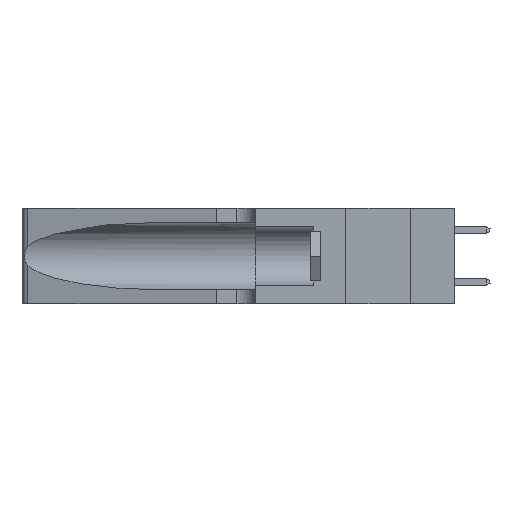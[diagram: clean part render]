
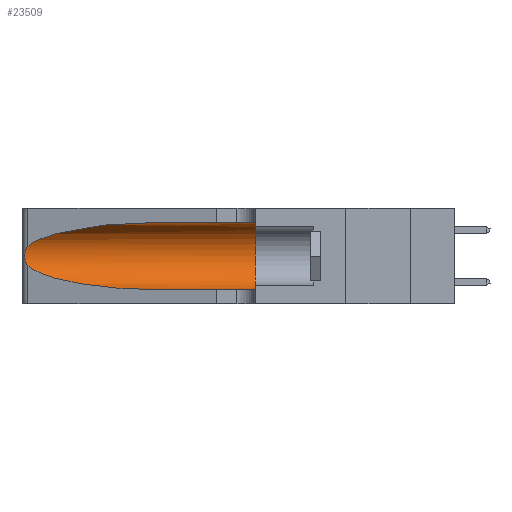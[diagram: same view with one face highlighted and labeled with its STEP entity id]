
A CAD part, left-side view. The second image highlights one B-rep face of the part: STEP entity #23509.
In plain terms, the highlighted cylindrical face has radius 3.308 mm (diameter 6.617 mm), a partial arc.
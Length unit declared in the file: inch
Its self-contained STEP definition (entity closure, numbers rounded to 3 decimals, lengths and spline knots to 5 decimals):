
#267 = VERTEX_POINT ( 'NONE', #5680 ) ;
#378 = VERTEX_POINT ( 'NONE', #12688 ) ;
#407 = CARTESIAN_POINT ( 'NONE',  ( 0.1305, 1.61858, 0.05475 ) ) ;
#580 = DIRECTION ( 'NONE',  ( 0., -1., 0. ) ) ;
#1451 = VERTEX_POINT ( 'NONE', #7885 ) ;
#1627 = CARTESIAN_POINT ( 'NONE',  ( 0.26075, 1.23896, 0.178 ) ) ;
#1999 =( BOUNDED_CURVE ( )  B_SPLINE_CURVE ( 3, ( #27865, #8334, #4212, #28052 ),
 .UNSPECIFIED., .F., .F. ) 
 B_SPLINE_CURVE_WITH_KNOTS ( ( 4, 4 ),
 ( 3.44316, 4.71239 ),
 .UNSPECIFIED. ) 
 CURVE ( )  GEOMETRIC_REPRESENTATION_ITEM ( )  RATIONAL_B_SPLINE_CURVE ( ( 1., 0.87, 0.87, 1. ) ) 
 REPRESENTATION_ITEM ( '' )  );
#2007 = CARTESIAN_POINT ( 'NONE',  ( 0.25639, 1.23184, 0.21858 ) ) ;
#2326 = DIRECTION ( 'NONE',  ( 0., 0., 1. ) ) ;
#2398 = LINE ( 'NONE', #3298, #26205 ) ;
#3022 = EDGE_CURVE ( 'NONE', #267, #16751, #1999, .T. ) ;
#3033 = EDGE_CURVE ( 'NONE', #16982, #267, #9717, .T. ) ;
#3298 = CARTESIAN_POINT ( 'NONE',  ( 0.1305, 1.61858, 0.31525 ) ) ;
#3930 = CARTESIAN_POINT ( 'NONE',  ( 0.25487, 1.22718, 0.14631 ) ) ;
#4212 = CARTESIAN_POINT ( 'NONE',  ( 0.18966, 0.96281, 0.05475 ) ) ;
#5383 = DIRECTION ( 'NONE',  ( 0., -1., 0. ) ) ;
#5680 = CARTESIAN_POINT ( 'NONE',  ( 0.25487, 1.22718, 0.14631 ) ) ;
#5920 = ORIENTED_EDGE ( 'NONE', *, *, #3022, .T. ) ;
#6170 = VERTEX_POINT ( 'NONE', #8930 ) ;
#6733 = CYLINDRICAL_SURFACE ( 'NONE', #8055, 0.13025 ) ;
#7602 =( BOUNDED_CURVE ( )  B_SPLINE_CURVE ( 3, ( #14610, #16617, #25393, #14525 ),
 .UNSPECIFIED., .F., .F. ) 
 B_SPLINE_CURVE_WITH_KNOTS ( ( 4, 4 ),
 ( 1.5708, 2.84003 ),
 .UNSPECIFIED. ) 
 CURVE ( )  GEOMETRIC_REPRESENTATION_ITEM ( )  RATIONAL_B_SPLINE_CURVE ( ( 1., 0.87, 0.87, 1. ) ) 
 REPRESENTATION_ITEM ( '' )  );
#7778 = FACE_OUTER_BOUND ( 'NONE', #12782, .T. ) ;
#7885 = CARTESIAN_POINT ( 'NONE',  ( 0.1305, 0.35, 0.31525 ) ) ;
#8055 = AXIS2_PLACEMENT_3D ( 'NONE', #9309, #580, #24467 ) ;
#8140 = CARTESIAN_POINT ( 'NONE',  ( 0.26017, 1.23833, 0.17102 ) ) ;
#8334 = CARTESIAN_POINT ( 'NONE',  ( 0.2373, 1.15595, 0.08982 ) ) ;
#8930 = CARTESIAN_POINT ( 'NONE',  ( 0.1305, 0.35, 0.05475 ) ) ;
#9309 = CARTESIAN_POINT ( 'NONE',  ( 0.1305, 1.61858, 0.185 ) ) ;
#9717 = B_SPLINE_CURVE_WITH_KNOTS ( 'NONE', 3,
 ( #12901, #10446, #2007, #25610, #12621, #14828, #21209, #1627, #8140, #23364, #16923, #25511, #12526, #3930 ),
 .UNSPECIFIED., .F., .F.,
 ( 4, 2, 2, 2, 2, 2, 4 ),
 ( 0., 0.00027, 0.00053, 0.00107, 0.0016, 0.00187, 0.00214 ),
 .UNSPECIFIED. ) ;
#10352 = EDGE_CURVE ( 'NONE', #1451, #6170, #19392, .T. ) ;
#10446 = CARTESIAN_POINT ( 'NONE',  ( 0.25555, 1.22994, 0.2215 ) ) ;
#11668 = AXIS2_PLACEMENT_3D ( 'NONE', #26992, #12390, #2326 ) ;
#12390 = DIRECTION ( 'NONE',  ( 0., 1., 0. ) ) ;
#12526 = CARTESIAN_POINT ( 'NONE',  ( 0.25555, 1.22993, 0.14849 ) ) ;
#12621 = CARTESIAN_POINT ( 'NONE',  ( 0.25854, 1.2359, 0.20912 ) ) ;
#12688 = CARTESIAN_POINT ( 'NONE',  ( 0.1305, 0.72297, 0.31525 ) ) ;
#12782 = EDGE_LOOP ( 'NONE', ( #23008, #19247, #5920, #17058, #26341, #27824 ) ) ;
#12901 = CARTESIAN_POINT ( 'NONE',  ( 0.25487, 1.22718, 0.22369 ) ) ;
#14026 = EDGE_CURVE ( 'NONE', #378, #1451, #2398, .T. ) ;
#14525 = CARTESIAN_POINT ( 'NONE',  ( 0.25487, 1.22718, 0.22369 ) ) ;
#14610 = CARTESIAN_POINT ( 'NONE',  ( 0.1305, 0.72297, 0.31525 ) ) ;
#14828 = CARTESIAN_POINT ( 'NONE',  ( 0.26018, 1.23835, 0.19895 ) ) ;
#15886 = EDGE_CURVE ( 'NONE', #378, #16982, #7602, .T. ) ;
#16617 = CARTESIAN_POINT ( 'NONE',  ( 0.18966, 0.96281, 0.31525 ) ) ;
#16751 = VERTEX_POINT ( 'NONE', #25997 ) ;
#16923 = CARTESIAN_POINT ( 'NONE',  ( 0.25789, 1.23486, 0.15765 ) ) ;
#16982 = VERTEX_POINT ( 'NONE', #24756 ) ;
#17058 = ORIENTED_EDGE ( 'NONE', *, *, #17961, .T. ) ;
#17936 = LINE ( 'NONE', #407, #25711 ) ;
#17961 = EDGE_CURVE ( 'NONE', #16751, #6170, #17936, .T. ) ;
#19247 = ORIENTED_EDGE ( 'NONE', *, *, #3033, .T. ) ;
#19392 = CIRCLE ( 'NONE', #11668, 0.13025 ) ;
#21209 = CARTESIAN_POINT ( 'NONE',  ( 0.26075, 1.23896, 0.19203 ) ) ;
#23008 = ORIENTED_EDGE ( 'NONE', *, *, #15886, .T. ) ;
#23364 = CARTESIAN_POINT ( 'NONE',  ( 0.25856, 1.23593, 0.16098 ) ) ;
#23509 = ADVANCED_FACE ( 'NONE', ( #7778 ), #6733, .F. ) ;
#24302 = DIRECTION ( 'NONE',  ( 0., -1., 0. ) ) ;
#24467 = DIRECTION ( 'NONE',  ( 0., 0., -1. ) ) ;
#24756 = CARTESIAN_POINT ( 'NONE',  ( 0.25487, 1.22718, 0.22369 ) ) ;
#25393 = CARTESIAN_POINT ( 'NONE',  ( 0.2373, 1.15595, 0.28018 ) ) ;
#25511 = CARTESIAN_POINT ( 'NONE',  ( 0.25639, 1.23186, 0.15144 ) ) ;
#25610 = CARTESIAN_POINT ( 'NONE',  ( 0.25787, 1.23484, 0.2124 ) ) ;
#25711 = VECTOR ( 'NONE', #24302, 39.37008 ) ;
#25997 = CARTESIAN_POINT ( 'NONE',  ( 0.1305, 0.72297, 0.05475 ) ) ;
#26205 = VECTOR ( 'NONE', #5383, 39.37008 ) ;
#26341 = ORIENTED_EDGE ( 'NONE', *, *, #10352, .F. ) ;
#26992 = CARTESIAN_POINT ( 'NONE',  ( 0.1305, 0.35, 0.185 ) ) ;
#27824 = ORIENTED_EDGE ( 'NONE', *, *, #14026, .F. ) ;
#27865 = CARTESIAN_POINT ( 'NONE',  ( 0.25487, 1.22718, 0.14631 ) ) ;
#28052 = CARTESIAN_POINT ( 'NONE',  ( 0.1305, 0.72297, 0.05475 ) ) ;
